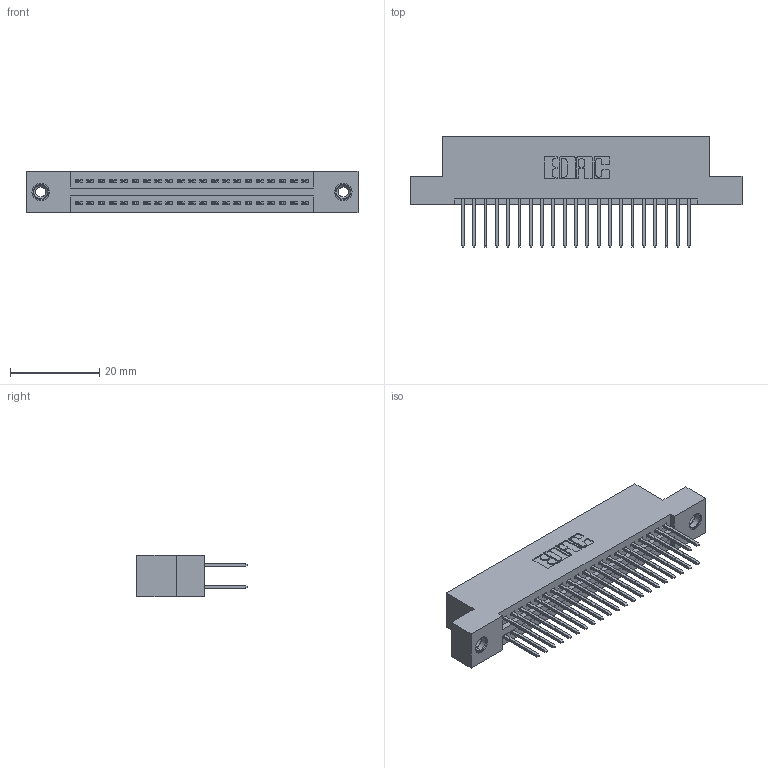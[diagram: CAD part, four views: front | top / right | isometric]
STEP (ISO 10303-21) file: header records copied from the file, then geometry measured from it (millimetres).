
FILE_DESCRIPTION (( 'STEP AP203' ), '1' );
FILE_NAME ('345-042-523-208.STEP', '2019-10-28T19:35:38', ( '' ), ( '' ), 'SwSTEP 2.0', 'SolidWorks 2016', '' );
FILE_SCHEMA (( 'CONFIG_CONTROL_DESIGN' ));
Length unit declared in the file: inch
Products named in the file (4): 345 Part_Flush Mounting Lugs - 0.156 Dia-TI; 345-250-001_345-250-003-102; 345-292-001_345-293-123; 345-042-523-208
Assembly tree (45 placements, depth 2):
  345-042-523-208
    345 Part_Flush Mounting Lugs - 0.156 Dia-TI
    345-292-001_345-293-123  x42
    345-250-001_345-250-003-102  x2
Bounding box: 74.55 x 24.82 x 9.4 mm (x, y, z)
Volume: 7126.4 mm3; surface area: 10526.9 mm2
Topology: 45 solids, 45 shells, 2286 faces, 6735 edges, 4426 vertices
Faces by surface type: plane 1498, cylinder 772, cone 12, torus 4
Entity records: 20508 total; most frequent: CARTESIAN_POINT 3439, ORIENTED_EDGE 3366, DIRECTION 3085, EDGE_CURVE 1683, LINE 1447, VECTOR 1447, VERTEX_POINT 1116, AXIS2_PLACEMENT_3D 819
